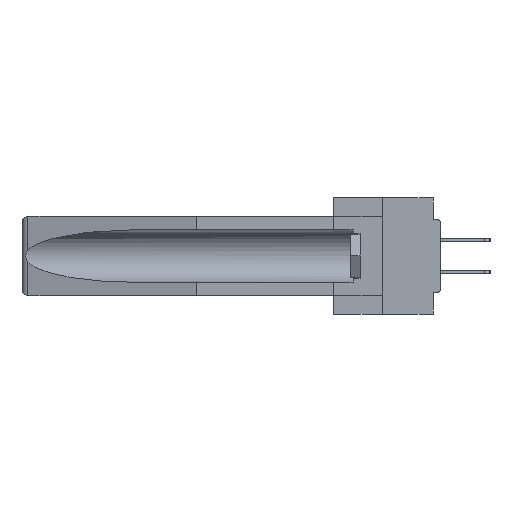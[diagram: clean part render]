
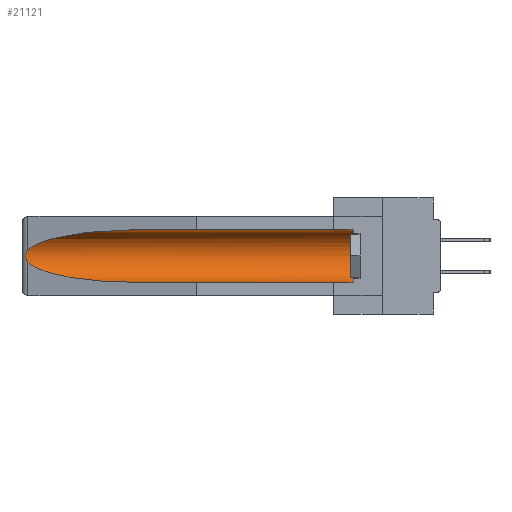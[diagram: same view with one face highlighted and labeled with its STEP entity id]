
A CAD part, left-side view. The second image highlights one B-rep face of the part: STEP entity #21121.
In plain terms, the highlighted cylindrical face has radius 2.857 mm (diameter 5.715 mm), a partial arc.
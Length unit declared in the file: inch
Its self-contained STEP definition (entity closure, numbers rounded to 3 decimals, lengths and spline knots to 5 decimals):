
#730 = VECTOR ( 'NONE', #20502, 39.37008 ) ;
#835 = ORIENTED_EDGE ( 'NONE', *, *, #33575, .T. ) ;
#1294 = CARTESIAN_POINT ( 'NONE',  ( 0.26537, 1.52718, -0.19328 ) ) ;
#1488 = CARTESIAN_POINT ( 'NONE',  ( 0.155, 1.07973, -0.284 ) ) ;
#2377 = CARTESIAN_POINT ( 'NONE',  ( 0.155, -0.30754, -0.059 ) ) ;
#3374 = CARTESIAN_POINT ( 'NONE',  ( 0.26655, 1.53094, -0.18657 ) ) ;
#3473 = CARTESIAN_POINT ( 'NONE',  ( 0.155, 1.07973, -0.059 ) ) ;
#3783 = AXIS2_PLACEMENT_3D ( 'NONE', #39896, #22919, #12264 ) ;
#3916 = CARTESIAN_POINT ( 'NONE',  ( 0.26537, 1.52718, -0.19328 ) ) ;
#5162 = ORIENTED_EDGE ( 'NONE', *, *, #24073, .T. ) ;
#6136 = VERTEX_POINT ( 'NONE', #38447 ) ;
#9047 = VECTOR ( 'NONE', #16477, 39.37008 ) ;
#10219 = CARTESIAN_POINT ( 'NONE',  ( 0.2673, 1.5327, -0.16383 ) ) ;
#10355 = CARTESIAN_POINT ( 'NONE',  ( 0.2675, 1.53308, -0.16763 ) ) ;
#10417 = ORIENTED_EDGE ( 'NONE', *, *, #33819, .T. ) ;
#12006 = B_SPLINE_CURVE_WITH_KNOTS ( 'NONE', 3,
 ( #21917, #20978, #31031, #10219, #10355, #34493, #13683, #3374, #15383, #1294 ),
 .UNSPECIFIED., .F., .F.,
 ( 4, 2, 2, 2, 4 ),
 ( 0., 0.00029, 0.00058, 0.00087, 0.00117 ),
 .UNSPECIFIED. ) ;
#12264 = DIRECTION ( 'NONE',  ( 0., 0., 1. ) ) ;
#12891 = AXIS2_PLACEMENT_3D ( 'NONE', #42846, #22264, #22108 ) ;
#13683 = CARTESIAN_POINT ( 'NONE',  ( 0.2673, 1.53269, -0.17917 ) ) ;
#13860 = VERTEX_POINT ( 'NONE', #26160 ) ;
#14108 = EDGE_CURVE ( 'NONE', #6136, #14830, #19721, .T. ) ;
#14830 = VERTEX_POINT ( 'NONE', #44417 ) ;
#15383 = CARTESIAN_POINT ( 'NONE',  ( 0.26597, 1.5296, -0.19026 ) ) ;
#16188 =( BOUNDED_CURVE ( )  B_SPLINE_CURVE ( 3, ( #3473, #16844, #16993, #20350 ),
 .UNSPECIFIED., .F., .F. ) 
 B_SPLINE_CURVE_WITH_KNOTS ( ( 4, 4 ),
 ( 4.71239, 6.08839 ),
 .UNSPECIFIED. ) 
 CURVE ( )  GEOMETRIC_REPRESENTATION_ITEM ( )  RATIONAL_B_SPLINE_CURVE ( ( 1., 0.848, 0.848, 1. ) ) 
 REPRESENTATION_ITEM ( '' )  );
#16477 = DIRECTION ( 'NONE',  ( 0., 1., 0. ) ) ;
#16844 = CARTESIAN_POINT ( 'NONE',  ( 0.21114, 1.30732, -0.059 ) ) ;
#16993 = CARTESIAN_POINT ( 'NONE',  ( 0.25451, 1.48313, -0.09465 ) ) ;
#18763 = CARTESIAN_POINT ( 'NONE',  ( 0.25451, 1.48313, -0.24835 ) ) ;
#19088 = FACE_OUTER_BOUND ( 'NONE', #40521, .T. ) ;
#19721 = LINE ( 'NONE', #43738, #730 ) ;
#20350 = CARTESIAN_POINT ( 'NONE',  ( 0.26537, 1.52718, -0.14972 ) ) ;
#20502 = DIRECTION ( 'NONE',  ( 0., 1., 0. ) ) ;
#20927 = LINE ( 'NONE', #2377, #9047 ) ;
#20978 = CARTESIAN_POINT ( 'NONE',  ( 0.26597, 1.52961, -0.15275 ) ) ;
#21121 = ADVANCED_FACE ( 'NONE', ( #19088 ), #34219, .F. ) ;
#21503 = VERTEX_POINT ( 'NONE', #28747 ) ;
#21917 = CARTESIAN_POINT ( 'NONE',  ( 0.26537, 1.52718, -0.14972 ) ) ;
#22108 = DIRECTION ( 'NONE',  ( 0., 0., 1. ) ) ;
#22264 = DIRECTION ( 'NONE',  ( 0., -1., 0. ) ) ;
#22919 = DIRECTION ( 'NONE',  ( 0., 1., 0. ) ) ;
#24073 = EDGE_CURVE ( 'NONE', #21503, #30161, #12006, .T. ) ;
#25005 = CIRCLE ( 'NONE', #12891, 0.1125 ) ;
#25230 = EDGE_CURVE ( 'NONE', #30161, #14830, #37585, .T. ) ;
#25300 = ORIENTED_EDGE ( 'NONE', *, *, #14108, .F. ) ;
#25881 = CARTESIAN_POINT ( 'NONE',  ( 0.155, 1.07973, -0.059 ) ) ;
#26160 = CARTESIAN_POINT ( 'NONE',  ( 0.155, 0.126, -0.059 ) ) ;
#26177 = EDGE_CURVE ( 'NONE', #13860, #31407, #20927, .T. ) ;
#28747 = CARTESIAN_POINT ( 'NONE',  ( 0.26537, 1.52718, -0.14972 ) ) ;
#30161 = VERTEX_POINT ( 'NONE', #3916 ) ;
#31031 = CARTESIAN_POINT ( 'NONE',  ( 0.26654, 1.53092, -0.15636 ) ) ;
#31407 = VERTEX_POINT ( 'NONE', #25881 ) ;
#31889 = ORIENTED_EDGE ( 'NONE', *, *, #26177, .T. ) ;
#33575 = EDGE_CURVE ( 'NONE', #31407, #21503, #16188, .T. ) ;
#33819 = EDGE_CURVE ( 'NONE', #6136, #13860, #25005, .T. ) ;
#34219 = CYLINDRICAL_SURFACE ( 'NONE', #3783, 0.1125 ) ;
#34493 = CARTESIAN_POINT ( 'NONE',  ( 0.2675, 1.53308, -0.17534 ) ) ;
#37585 =( BOUNDED_CURVE ( )  B_SPLINE_CURVE ( 3, ( #40733, #18763, #39701, #1488 ),
 .UNSPECIFIED., .F., .F. ) 
 B_SPLINE_CURVE_WITH_KNOTS ( ( 4, 4 ),
 ( 0.1948, 1.5708 ),
 .UNSPECIFIED. ) 
 CURVE ( )  GEOMETRIC_REPRESENTATION_ITEM ( )  RATIONAL_B_SPLINE_CURVE ( ( 1., 0.848, 0.848, 1. ) ) 
 REPRESENTATION_ITEM ( '' )  );
#38447 = CARTESIAN_POINT ( 'NONE',  ( 0.155, 0.126, -0.284 ) ) ;
#39701 = CARTESIAN_POINT ( 'NONE',  ( 0.21114, 1.30732, -0.284 ) ) ;
#39896 = CARTESIAN_POINT ( 'NONE',  ( 0.155, -0.30754, -0.1715 ) ) ;
#40521 = EDGE_LOOP ( 'NONE', ( #835, #5162, #44117, #25300, #10417, #31889 ) ) ;
#40733 = CARTESIAN_POINT ( 'NONE',  ( 0.26537, 1.52718, -0.19328 ) ) ;
#42846 = CARTESIAN_POINT ( 'NONE',  ( 0.155, 0.126, -0.1715 ) ) ;
#43738 = CARTESIAN_POINT ( 'NONE',  ( 0.155, -0.30754, -0.284 ) ) ;
#44117 = ORIENTED_EDGE ( 'NONE', *, *, #25230, .T. ) ;
#44417 = CARTESIAN_POINT ( 'NONE',  ( 0.155, 1.07973, -0.284 ) ) ;
